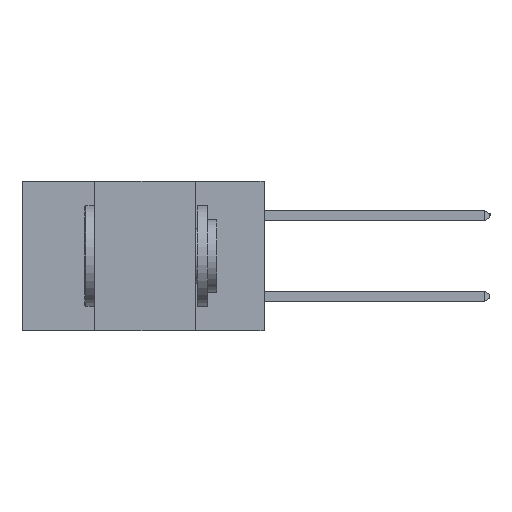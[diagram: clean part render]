
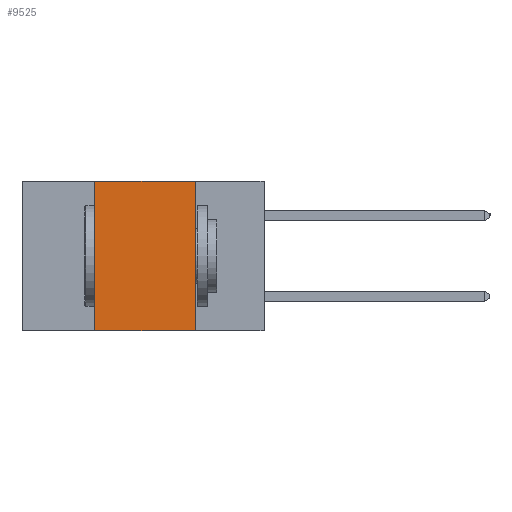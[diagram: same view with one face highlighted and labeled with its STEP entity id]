
A CAD part, left-side view. The second image highlights one B-rep face of the part: STEP entity #9525.
In plain terms, the highlighted planar face has unit normal (-1, 0, 0).
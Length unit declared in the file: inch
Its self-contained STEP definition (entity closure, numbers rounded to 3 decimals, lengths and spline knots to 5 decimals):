
#188 = DIRECTION ( 'NONE',  ( 0., -1., 0. ) ) ;
#582 = DIRECTION ( 'NONE',  ( 0., -1., 0. ) ) ;
#1743 = FACE_OUTER_BOUND ( 'NONE', #8194, .T. ) ;
#2972 = EDGE_CURVE ( 'NONE', #18399, #3556, #14501, .T. ) ;
#3556 = VERTEX_POINT ( 'NONE', #16889 ) ;
#3736 = VECTOR ( 'NONE', #188, 39.37008 ) ;
#4046 = CARTESIAN_POINT ( 'NONE',  ( 0., 0.17, -0.37 ) ) ;
#4141 = CARTESIAN_POINT ( 'NONE',  ( 0., 0.42, -0.37 ) ) ;
#4557 = EDGE_CURVE ( 'NONE', #18399, #17358, #17040, .T. ) ;
#4637 = CARTESIAN_POINT ( 'NONE',  ( 0., 0.6, 0. ) ) ;
#4740 = LINE ( 'NONE', #7834, #13695 ) ;
#4995 = AXIS2_PLACEMENT_3D ( 'NONE', #4637, #10398, #16144 ) ;
#5371 = CARTESIAN_POINT ( 'NONE',  ( 0., 0.42, -0.37 ) ) ;
#6805 = ORIENTED_EDGE ( 'NONE', *, *, #8140, .F. ) ;
#7300 = VECTOR ( 'NONE', #15558, 39.37008 ) ;
#7339 = CARTESIAN_POINT ( 'NONE',  ( 0., 0.6, -0.37 ) ) ;
#7469 = CARTESIAN_POINT ( 'NONE',  ( 0., 0.42, 0. ) ) ;
#7799 = CARTESIAN_POINT ( 'NONE',  ( 0., 0.17, 0. ) ) ;
#7834 = CARTESIAN_POINT ( 'NONE',  ( 0., 0.6, 0. ) ) ;
#8140 = EDGE_CURVE ( 'NONE', #17358, #14314, #4740, .T. ) ;
#8194 = EDGE_LOOP ( 'NONE', ( #14619, #6805, #15333, #18008 ) ) ;
#9525 = ADVANCED_FACE ( 'NONE', ( #1743 ), #17546, .F. ) ;
#10398 = DIRECTION ( 'NONE',  ( 1., 0., 0. ) ) ;
#13695 = VECTOR ( 'NONE', #582, 39.37008 ) ;
#14314 = VERTEX_POINT ( 'NONE', #7799 ) ;
#14501 = LINE ( 'NONE', #7339, #3736 ) ;
#14619 = ORIENTED_EDGE ( 'NONE', *, *, #16294, .F. ) ;
#15333 = ORIENTED_EDGE ( 'NONE', *, *, #4557, .F. ) ;
#15435 = DIRECTION ( 'NONE',  ( 0., 0., 1. ) ) ;
#15558 = DIRECTION ( 'NONE',  ( 0., 0., -1. ) ) ;
#16144 = DIRECTION ( 'NONE',  ( 0., 0., -1. ) ) ;
#16294 = EDGE_CURVE ( 'NONE', #14314, #3556, #16953, .T. ) ;
#16723 = VECTOR ( 'NONE', #15435, 39.37008 ) ;
#16889 = CARTESIAN_POINT ( 'NONE',  ( 0., 0.17, -0.37 ) ) ;
#16953 = LINE ( 'NONE', #4046, #7300 ) ;
#17040 = LINE ( 'NONE', #4141, #16723 ) ;
#17358 = VERTEX_POINT ( 'NONE', #7469 ) ;
#17546 = PLANE ( 'NONE',  #4995 ) ;
#18008 = ORIENTED_EDGE ( 'NONE', *, *, #2972, .T. ) ;
#18399 = VERTEX_POINT ( 'NONE', #5371 ) ;
